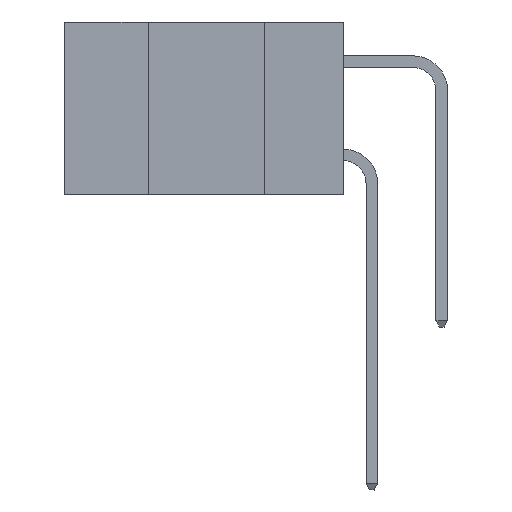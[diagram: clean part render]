
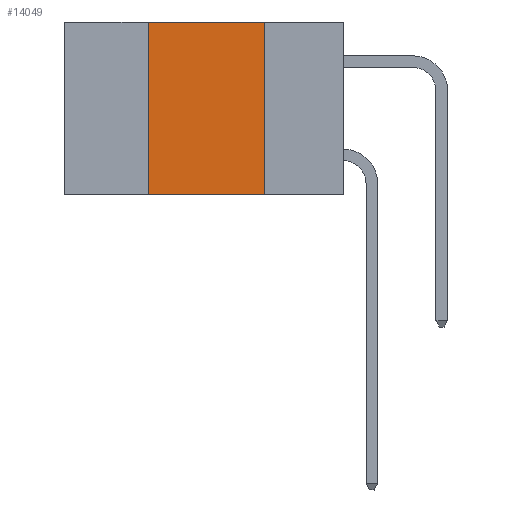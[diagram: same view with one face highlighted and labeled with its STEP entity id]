
A CAD part, left-side view. The second image highlights one B-rep face of the part: STEP entity #14049.
In plain terms, the highlighted planar face has unit normal (-1, 0, 0).
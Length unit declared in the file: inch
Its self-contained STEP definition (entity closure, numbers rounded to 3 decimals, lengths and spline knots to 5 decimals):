
#373 = CARTESIAN_POINT ( 'NONE',  ( 0., 0.17, -0.37 ) ) ;
#538 = VECTOR ( 'NONE', #9678, 39.37008 ) ;
#1527 = EDGE_LOOP ( 'NONE', ( #1793, #6809, #8235, #8756 ) ) ;
#1566 = EDGE_CURVE ( 'NONE', #10894, #10350, #4393, .T. ) ;
#1793 = ORIENTED_EDGE ( 'NONE', *, *, #4123, .F. ) ;
#1929 = VECTOR ( 'NONE', #2687, 39.37008 ) ;
#2687 = DIRECTION ( 'NONE',  ( 0., -1., 0. ) ) ;
#3254 = CARTESIAN_POINT ( 'NONE',  ( 0., 0.6, 0. ) ) ;
#4123 = EDGE_CURVE ( 'NONE', #10350, #4866, #5841, .T. ) ;
#4393 = LINE ( 'NONE', #3254, #538 ) ;
#4430 = DIRECTION ( 'NONE',  ( 0., 0., 1. ) ) ;
#4866 = VERTEX_POINT ( 'NONE', #7045 ) ;
#5759 = DIRECTION ( 'NONE',  ( 0., 0., -1. ) ) ;
#5841 = LINE ( 'NONE', #373, #7491 ) ;
#6112 = EDGE_CURVE ( 'NONE', #8554, #4866, #15945, .T. ) ;
#6809 = ORIENTED_EDGE ( 'NONE', *, *, #1566, .F. ) ;
#7014 = VECTOR ( 'NONE', #4430, 39.37008 ) ;
#7045 = CARTESIAN_POINT ( 'NONE',  ( 0., 0.17, -0.37 ) ) ;
#7125 = CARTESIAN_POINT ( 'NONE',  ( 0., 0.6, 0. ) ) ;
#7284 = AXIS2_PLACEMENT_3D ( 'NONE', #7125, #12156, #8426 ) ;
#7491 = VECTOR ( 'NONE', #5759, 39.37008 ) ;
#7625 = CARTESIAN_POINT ( 'NONE',  ( 0., 0.17, 0. ) ) ;
#8235 = ORIENTED_EDGE ( 'NONE', *, *, #14099, .F. ) ;
#8253 = FACE_OUTER_BOUND ( 'NONE', #1527, .T. ) ;
#8426 = DIRECTION ( 'NONE',  ( 0., 0., -1. ) ) ;
#8554 = VERTEX_POINT ( 'NONE', #16033 ) ;
#8756 = ORIENTED_EDGE ( 'NONE', *, *, #6112, .T. ) ;
#9678 = DIRECTION ( 'NONE',  ( 0., -1., 0. ) ) ;
#10350 = VERTEX_POINT ( 'NONE', #7625 ) ;
#10894 = VERTEX_POINT ( 'NONE', #15477 ) ;
#12156 = DIRECTION ( 'NONE',  ( 1., 0., 0. ) ) ;
#12504 = PLANE ( 'NONE',  #7284 ) ;
#14049 = ADVANCED_FACE ( 'NONE', ( #8253 ), #12504, .F. ) ;
#14099 = EDGE_CURVE ( 'NONE', #8554, #10894, #14916, .T. ) ;
#14560 = CARTESIAN_POINT ( 'NONE',  ( 0., 0.6, -0.37 ) ) ;
#14916 = LINE ( 'NONE', #16310, #7014 ) ;
#15477 = CARTESIAN_POINT ( 'NONE',  ( 0., 0.42, 0. ) ) ;
#15945 = LINE ( 'NONE', #14560, #1929 ) ;
#16033 = CARTESIAN_POINT ( 'NONE',  ( 0., 0.42, -0.37 ) ) ;
#16310 = CARTESIAN_POINT ( 'NONE',  ( 0., 0.42, -0.37 ) ) ;
